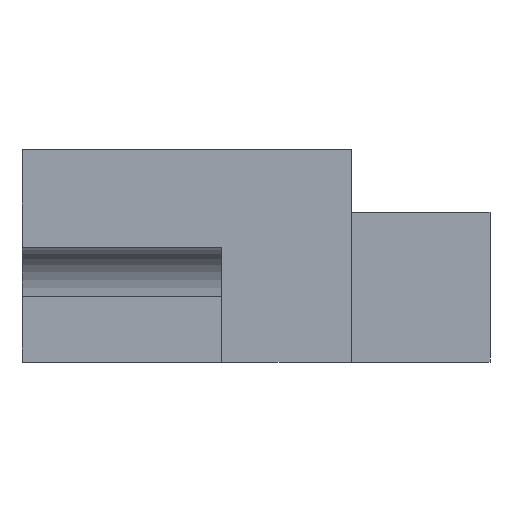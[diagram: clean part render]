
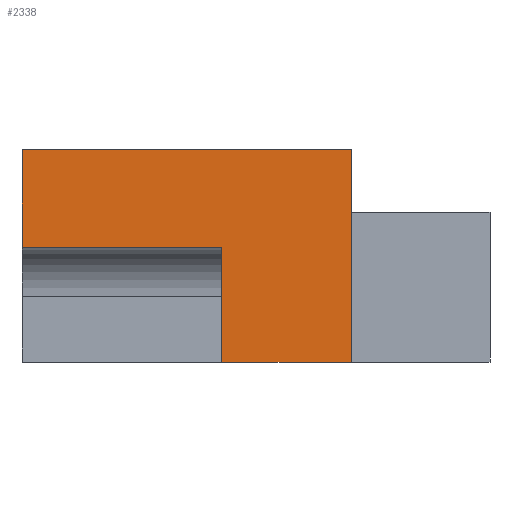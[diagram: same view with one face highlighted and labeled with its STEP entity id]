
A CAD part, left-side view. The second image highlights one B-rep face of the part: STEP entity #2338.
In plain terms, the highlighted planar face has unit normal (-1, 0, 0).
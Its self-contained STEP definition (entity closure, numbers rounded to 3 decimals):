
#202 = EDGE_CURVE ( 'NONE', #1689, #495, #3795, .T. ) ;
#294 = LINE ( 'NONE', #16578, #19465 ) ;
#401 = DIRECTION ( 'NONE',  ( 0., 1., 0. ) ) ;
#495 = VERTEX_POINT ( 'NONE', #6928 ) ;
#536 = VECTOR ( 'NONE', #7954, 1000. ) ;
#721 = CARTESIAN_POINT ( 'NONE',  ( 0., 11.506, 0. ) ) ;
#1689 = VERTEX_POINT ( 'NONE', #18115 ) ;
#2238 = VECTOR ( 'NONE', #13573, 1000. ) ;
#2266 = EDGE_CURVE ( 'NONE', #5704, #20155, #4717, .T. ) ;
#2338 = ADVANCED_FACE ( 'NONE', ( #7805 ), #16911, .F. ) ;
#2603 = ORIENTED_EDGE ( 'NONE', *, *, #8170, .F. ) ;
#2967 = AXIS2_PLACEMENT_3D ( 'NONE', #15699, #7894, #3882 ) ;
#3795 = LINE ( 'NONE', #5742, #20675 ) ;
#3882 = DIRECTION ( 'NONE',  ( 0., 0., -1. ) ) ;
#4086 = DIRECTION ( 'NONE',  ( 0., 0., -1. ) ) ;
#4462 = EDGE_LOOP ( 'NONE', ( #19614, #20192, #14601, #17707, #5827, #2603 ) ) ;
#4717 = LINE ( 'NONE', #13867, #13397 ) ;
#4971 = VECTOR ( 'NONE', #16527, 1000. ) ;
#5704 = VERTEX_POINT ( 'NONE', #12032 ) ;
#5742 = CARTESIAN_POINT ( 'NONE',  ( 0., 20.955, -13.487 ) ) ;
#5827 = ORIENTED_EDGE ( 'NONE', *, *, #20648, .F. ) ;
#6444 = CARTESIAN_POINT ( 'NONE',  ( 0., 8.255, -13.487 ) ) ;
#6928 = CARTESIAN_POINT ( 'NONE',  ( 0., 20.955, 0. ) ) ;
#7805 = FACE_OUTER_BOUND ( 'NONE', #4462, .T. ) ;
#7894 = DIRECTION ( 'NONE',  ( 1., 0., 0. ) ) ;
#7954 = DIRECTION ( 'NONE',  ( 0., 0., 1. ) ) ;
#8170 = EDGE_CURVE ( 'NONE', #8967, #20031, #19181, .T. ) ;
#8967 = VERTEX_POINT ( 'NONE', #17282 ) ;
#9327 = LINE ( 'NONE', #9647, #4971 ) ;
#9647 = CARTESIAN_POINT ( 'NONE',  ( 0., 8.255, -6.172 ) ) ;
#10105 = CARTESIAN_POINT ( 'NONE',  ( 0., 0., -13.487 ) ) ;
#10750 = EDGE_CURVE ( 'NONE', #495, #5704, #15035, .T. ) ;
#12032 = CARTESIAN_POINT ( 'NONE',  ( 0., 0., 0. ) ) ;
#13397 = VECTOR ( 'NONE', #4086, 1000. ) ;
#13573 = DIRECTION ( 'NONE',  ( 0., -1., 0. ) ) ;
#13867 = CARTESIAN_POINT ( 'NONE',  ( 0., 0., 0. ) ) ;
#14601 = ORIENTED_EDGE ( 'NONE', *, *, #10750, .F. ) ;
#14942 = EDGE_CURVE ( 'NONE', #20155, #8967, #294, .T. ) ;
#15035 = LINE ( 'NONE', #721, #2238 ) ;
#15388 = DIRECTION ( 'NONE',  ( 0., 0., 1. ) ) ;
#15699 = CARTESIAN_POINT ( 'NONE',  ( 0., 0., 0. ) ) ;
#16527 = DIRECTION ( 'NONE',  ( 0., 1., 0. ) ) ;
#16578 = CARTESIAN_POINT ( 'NONE',  ( 0., -8.814, -13.487 ) ) ;
#16911 = PLANE ( 'NONE',  #2967 ) ;
#17282 = CARTESIAN_POINT ( 'NONE',  ( 0., 8.255, -13.487 ) ) ;
#17707 = ORIENTED_EDGE ( 'NONE', *, *, #202, .F. ) ;
#18032 = CARTESIAN_POINT ( 'NONE',  ( 0., 8.255, -6.172 ) ) ;
#18115 = CARTESIAN_POINT ( 'NONE',  ( 0., 20.955, -6.172 ) ) ;
#19181 = LINE ( 'NONE', #6444, #536 ) ;
#19465 = VECTOR ( 'NONE', #401, 1000. ) ;
#19614 = ORIENTED_EDGE ( 'NONE', *, *, #14942, .F. ) ;
#20031 = VERTEX_POINT ( 'NONE', #18032 ) ;
#20155 = VERTEX_POINT ( 'NONE', #10105 ) ;
#20192 = ORIENTED_EDGE ( 'NONE', *, *, #2266, .F. ) ;
#20648 = EDGE_CURVE ( 'NONE', #20031, #1689, #9327, .T. ) ;
#20675 = VECTOR ( 'NONE', #15388, 1000. ) ;
